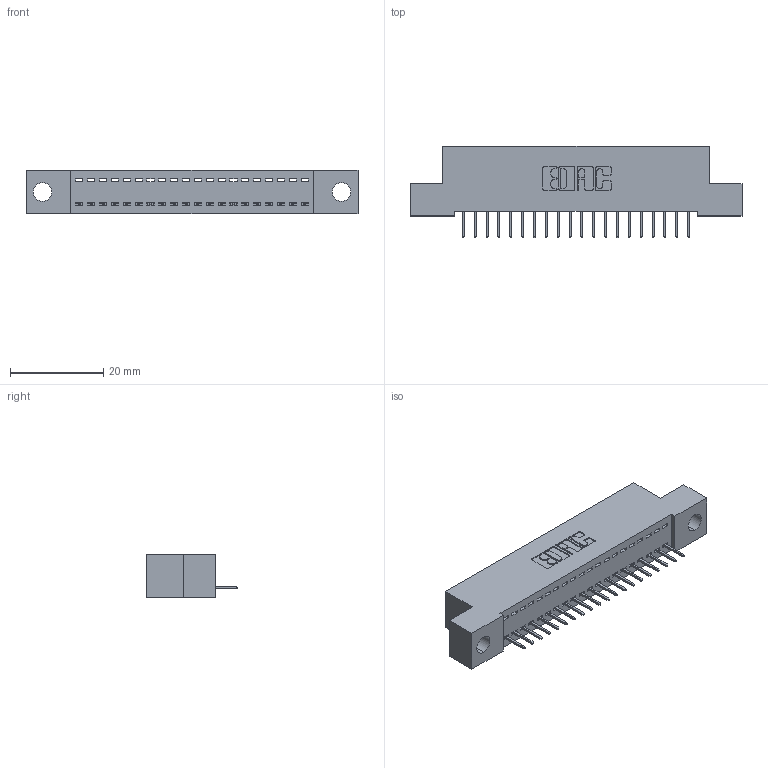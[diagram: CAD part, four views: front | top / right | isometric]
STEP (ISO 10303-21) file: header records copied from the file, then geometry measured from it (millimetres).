
FILE_DESCRIPTION (( 'STEP AP203' ), '1' );
FILE_NAME ('342-020-524-104.STEP', '2018-08-10T22:49:09', ( '' ), ( '' ), 'SwSTEP 2.0', 'SolidWorks 2016', '' );
FILE_SCHEMA (( 'CONFIG_CONTROL_DESIGN' ));
Length unit declared in the file: inch
Products named in the file (3): 342 Part_.156 TH; 345-292-001_345-293-124; 342-020-524-104
Assembly tree (21 placements, depth 2):
  342-020-524-104
    342 Part_.156 TH
    345-292-001_345-293-124  x20
Bounding box: 71.12 x 19.69 x 9.4 mm (x, y, z)
Volume: 5988.7 mm3; surface area: 7956.8 mm2
Topology: 21 solids, 21 shells, 1350 faces, 3899 edges, 2518 vertices
Faces by surface type: plane 1026, cylinder 324
Entity records: 15017 total; most frequent: CARTESIAN_POINT 2598, ORIENTED_EDGE 2554, DIRECTION 2237, EDGE_CURVE 1277, VECTOR 1153, LINE 1153, VERTEX_POINT 846, AXIS2_PLACEMENT_3D 542
